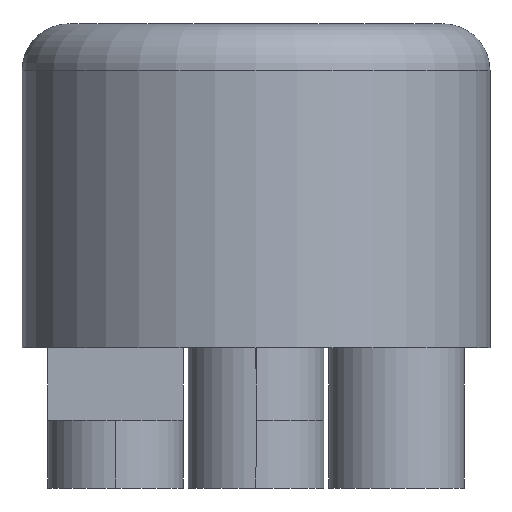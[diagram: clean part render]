
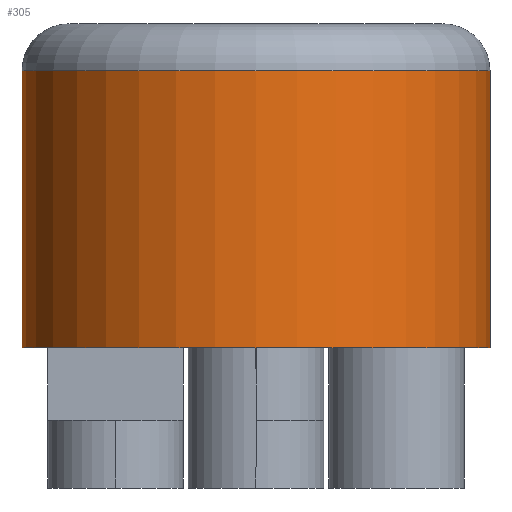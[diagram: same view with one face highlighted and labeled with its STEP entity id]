
A CAD part, front view. The second image highlights one B-rep face of the part: STEP entity #305.
In plain terms, the highlighted cylindrical face has radius 25 mm (diameter 50 mm), a partial arc.
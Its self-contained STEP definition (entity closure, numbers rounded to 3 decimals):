
#183 = CARTESIAN_POINT ( 'NONE',  ( 0., 0., 17.3 ) ) ;
#187 = DIRECTION ( 'NONE',  ( 0., 0., -1. ) ) ;
#206 = CARTESIAN_POINT ( 'NONE',  ( 25., 0., 17.3 ) ) ;
#213 = CIRCLE ( 'NONE', #550, 25. ) ;
#237 = CIRCLE ( 'NONE', #585, 25. ) ;
#242 = DIRECTION ( 'NONE',  ( -1., 0., 0. ) ) ;
#259 = DIRECTION ( 'NONE',  ( 0., 0., -1. ) ) ;
#281 = CARTESIAN_POINT ( 'NONE',  ( -25., 0., 17.3 ) ) ;
#284 = DIRECTION ( 'NONE',  ( 0., 0., -1. ) ) ;
#291 = VECTOR ( 'NONE', #284, 1000. ) ;
#296 = LINE ( 'NONE', #281, #291 ) ;
#297 = VECTOR ( 'NONE', #259, 1000. ) ;
#302 = LINE ( 'NONE', #206, #297 ) ;
#305 = ADVANCED_FACE ( 'NONE', ( #428 ), #419, .T. ) ;
#419 = CYLINDRICAL_SURFACE ( 'NONE', #700, 25. ) ;
#428 = FACE_OUTER_BOUND ( 'NONE', #1133, .T. ) ;
#497 = ORIENTED_EDGE ( 'NONE', *, *, #919, .T. ) ;
#550 = AXIS2_PLACEMENT_3D ( 'NONE', #828, #830, #834 ) ;
#559 = CARTESIAN_POINT ( 'NONE',  ( 0., 0., -17.3 ) ) ;
#563 = DIRECTION ( 'NONE',  ( 0., 0., -1. ) ) ;
#568 = DIRECTION ( 'NONE',  ( -1., 0., 0. ) ) ;
#585 = AXIS2_PLACEMENT_3D ( 'NONE', #559, #563, #568 ) ;
#697 = ORIENTED_EDGE ( 'NONE', *, *, #829, .F. ) ;
#700 = AXIS2_PLACEMENT_3D ( 'NONE', #183, #187, #242 ) ;
#705 = VERTEX_POINT ( 'NONE', #1131 ) ;
#720 = ORIENTED_EDGE ( 'NONE', *, *, #890, .F. ) ;
#750 = VERTEX_POINT ( 'NONE', #1119 ) ;
#757 = CARTESIAN_POINT ( 'NONE',  ( -25., 0., 12.3 ) ) ;
#828 = CARTESIAN_POINT ( 'NONE',  ( 0., 0., 12.3 ) ) ;
#829 = EDGE_CURVE ( 'NONE', #750, #1037, #302, .T. ) ;
#830 = DIRECTION ( 'NONE',  ( 0., 0., -1. ) ) ;
#832 = EDGE_CURVE ( 'NONE', #917, #705, #296, .T. ) ;
#834 = DIRECTION ( 'NONE',  ( 1., 0., 0. ) ) ;
#889 = CARTESIAN_POINT ( 'NONE',  ( 25., 0., -17.3 ) ) ;
#890 = EDGE_CURVE ( 'NONE', #1037, #705, #237, .T. ) ;
#897 = ORIENTED_EDGE ( 'NONE', *, *, #832, .T. ) ;
#917 = VERTEX_POINT ( 'NONE', #757 ) ;
#919 = EDGE_CURVE ( 'NONE', #750, #917, #213, .T. ) ;
#1037 = VERTEX_POINT ( 'NONE', #889 ) ;
#1119 = CARTESIAN_POINT ( 'NONE',  ( 25., 0., 12.3 ) ) ;
#1131 = CARTESIAN_POINT ( 'NONE',  ( -25., 0., -17.3 ) ) ;
#1133 = EDGE_LOOP ( 'NONE', ( #697, #497, #897, #720 ) ) ;
